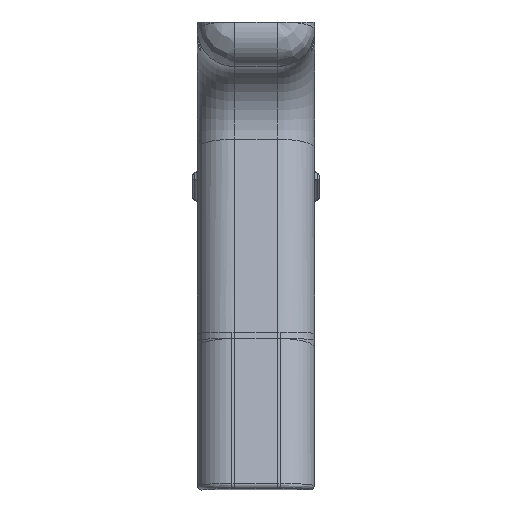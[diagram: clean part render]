
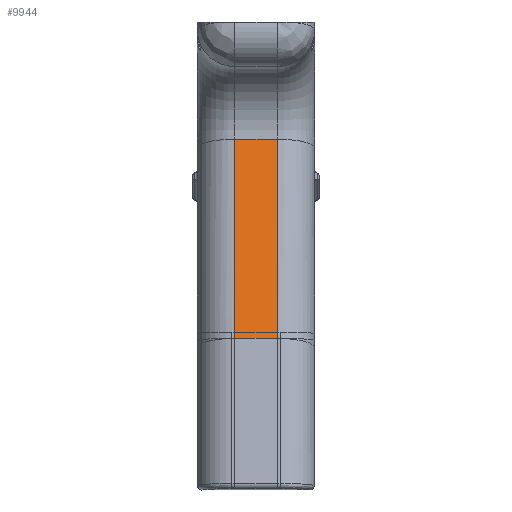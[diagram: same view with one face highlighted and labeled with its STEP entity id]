
A CAD part, front view. The second image highlights one B-rep face of the part: STEP entity #9944.
In plain terms, the highlighted face is planar.
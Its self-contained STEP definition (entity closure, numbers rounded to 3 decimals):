
#936=FACE_OUTER_BOUND('',#1505,.T.);
#1505=EDGE_LOOP('',(#8096,#8097,#8098,#8099));
#2162=LINE('',#16690,#3029);
#2316=LINE('',#17535,#3183);
#2317=LINE('',#17538,#3184);
#2318=LINE('',#17539,#3185);
#3029=VECTOR('',#12407,10.);
#3183=VECTOR('',#12807,10.);
#3184=VECTOR('',#12810,10.);
#3185=VECTOR('',#12811,10.);
#4385=VERTEX_POINT('',#16686);
#4386=VERTEX_POINT('',#16688);
#4521=VERTEX_POINT('',#17513);
#4524=VERTEX_POINT('',#17537);
#5576=EDGE_CURVE('',#4385,#4386,#2162,.T.);
#5800=EDGE_CURVE('',#4385,#4521,#2316,.T.);
#5801=EDGE_CURVE('',#4524,#4386,#2317,.T.);
#5802=EDGE_CURVE('',#4521,#4524,#2318,.T.);
#8096=ORIENTED_EDGE('',*,*,#5801,.F.);
#8097=ORIENTED_EDGE('',*,*,#5802,.F.);
#8098=ORIENTED_EDGE('',*,*,#5800,.F.);
#8099=ORIENTED_EDGE('',*,*,#5576,.T.);
#9525=PLANE('',#10788);
#9944=ADVANCED_FACE('',(#936),#9525,.T.);
#10788=AXIS2_PLACEMENT_3D('',#17536,#12808,#12809);
#12407=DIRECTION('',(0.,-0.249,0.969));
#12807=DIRECTION('',(-1.,0.,0.));
#12808=DIRECTION('center_axis',(0.,-0.969,
-0.249));
#12809=DIRECTION('ref_axis',(0.,-0.249,0.969));
#12810=DIRECTION('',(1.,0.,0.));
#12811=DIRECTION('',(0.,-0.249,0.969));
#16686=CARTESIAN_POINT('',(13.45,-71.634,19.877));
#16688=CARTESIAN_POINT('',(13.45,-83.628,66.536));
#16690=CARTESIAN_POINT('',(13.45,-83.554,66.245));
#17513=CARTESIAN_POINT('',(3.45,-71.634,19.877));
#17535=CARTESIAN_POINT('',(22.175,-71.634,19.877));
#17536=CARTESIAN_POINT('Origin',(22.175,-71.634,19.877));
#17537=CARTESIAN_POINT('',(3.45,-83.628,66.536));
#17538=CARTESIAN_POINT('',(22.175,-83.628,66.536));
#17539=CARTESIAN_POINT('',(3.45,-83.554,66.245));
